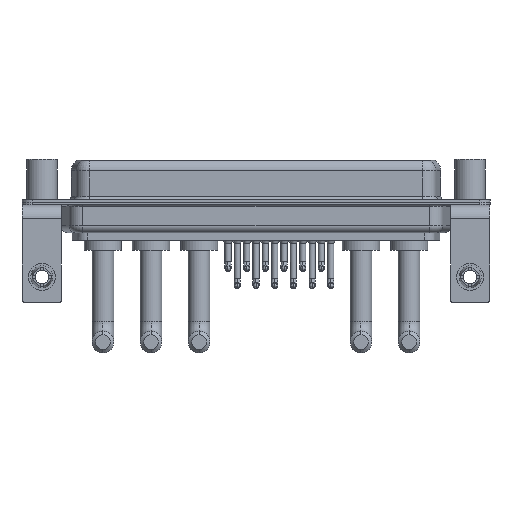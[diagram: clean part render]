
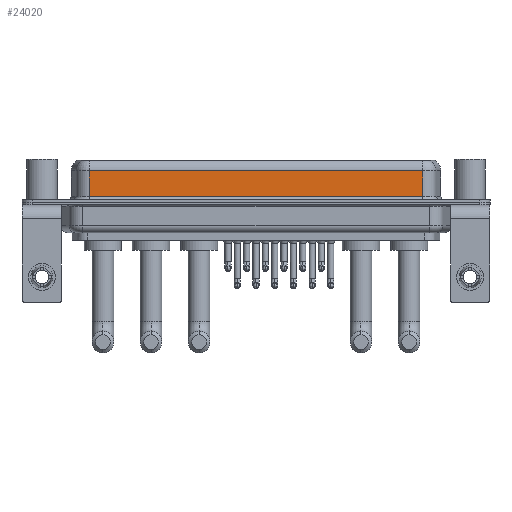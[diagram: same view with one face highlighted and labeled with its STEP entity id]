
A CAD part, front view. The second image highlights one B-rep face of the part: STEP entity #24020.
In plain terms, the highlighted planar face has unit normal (0, -1, 0).
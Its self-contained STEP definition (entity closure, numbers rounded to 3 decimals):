
#1425 = VECTOR ( 'NONE', #15554, 1000. ) ;
#1482 = FACE_OUTER_BOUND ( 'NONE', #6186, .T. ) ;
#1599 = DIRECTION ( 'NONE',  ( 0., 1., 0. ) ) ;
#2480 = DIRECTION ( 'NONE',  ( 0., 0., -1. ) ) ;
#3092 = PLANE ( 'NONE',  #14159 ) ;
#3195 = CARTESIAN_POINT ( 'NONE',  ( 56.462, -3.95, 0.9 ) ) ;
#4765 = ORIENTED_EDGE ( 'NONE', *, *, #6075, .T. ) ;
#6075 = EDGE_CURVE ( 'NONE', #21098, #19340, #20805, .T. ) ;
#6186 = EDGE_LOOP ( 'NONE', ( #17317, #18696, #10614, #4765 ) ) ;
#7593 = CARTESIAN_POINT ( 'NONE',  ( 56.462, -3.95, 4.65 ) ) ;
#7982 = DIRECTION ( 'NONE',  ( 1., 0., 0. ) ) ;
#10011 = LINE ( 'NONE', #13826, #1425 ) ;
#10238 = VECTOR ( 'NONE', #2480, 1000. ) ;
#10355 = VERTEX_POINT ( 'NONE', #22588 ) ;
#10614 = ORIENTED_EDGE ( 'NONE', *, *, #17826, .T. ) ;
#11229 = VERTEX_POINT ( 'NONE', #22522 ) ;
#11424 = DIRECTION ( 'NONE',  ( -1., 0., 0. ) ) ;
#11810 = CARTESIAN_POINT ( 'NONE',  ( 56.462, -3.95, 0.9 ) ) ;
#12863 = VECTOR ( 'NONE', #11424, 1000. ) ;
#12939 = EDGE_CURVE ( 'NONE', #11229, #19340, #10011, .T. ) ;
#13030 = LINE ( 'NONE', #7593, #12863 ) ;
#13688 = LINE ( 'NONE', #15545, #10238 ) ;
#13826 = CARTESIAN_POINT ( 'NONE',  ( 56.462, -3.95, 6.4 ) ) ;
#14159 = AXIS2_PLACEMENT_3D ( 'NONE', #18457, #1599, #16505 ) ;
#15135 = EDGE_CURVE ( 'NONE', #11229, #10355, #13030, .T. ) ;
#15545 = CARTESIAN_POINT ( 'NONE',  ( 7.038, -3.95, 6.4 ) ) ;
#15554 = DIRECTION ( 'NONE',  ( 0., 0., -1. ) ) ;
#16505 = DIRECTION ( 'NONE',  ( 0., 0., 1. ) ) ;
#17317 = ORIENTED_EDGE ( 'NONE', *, *, #12939, .F. ) ;
#17826 = EDGE_CURVE ( 'NONE', #10355, #21098, #13688, .T. ) ;
#18356 = VECTOR ( 'NONE', #7982, 1000. ) ;
#18457 = CARTESIAN_POINT ( 'NONE',  ( 56.462, -3.95, 6.4 ) ) ;
#18696 = ORIENTED_EDGE ( 'NONE', *, *, #15135, .T. ) ;
#19340 = VERTEX_POINT ( 'NONE', #3195 ) ;
#20805 = LINE ( 'NONE', #11810, #18356 ) ;
#21098 = VERTEX_POINT ( 'NONE', #22302 ) ;
#22302 = CARTESIAN_POINT ( 'NONE',  ( 7.038, -3.95, 0.9 ) ) ;
#22522 = CARTESIAN_POINT ( 'NONE',  ( 56.462, -3.95, 4.65 ) ) ;
#22588 = CARTESIAN_POINT ( 'NONE',  ( 7.038, -3.95, 4.65 ) ) ;
#24020 = ADVANCED_FACE ( 'NONE', ( #1482 ), #3092, .F. ) ;
